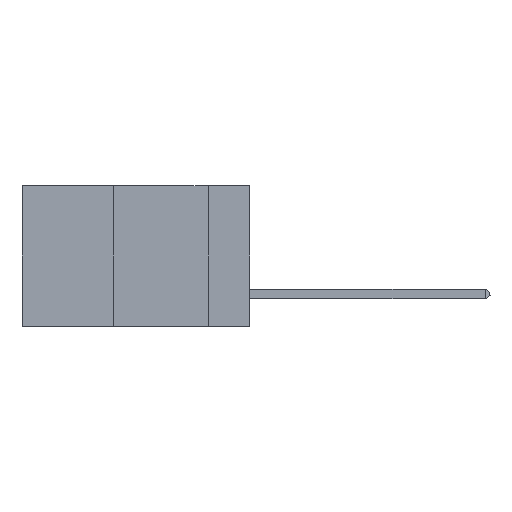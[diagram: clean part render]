
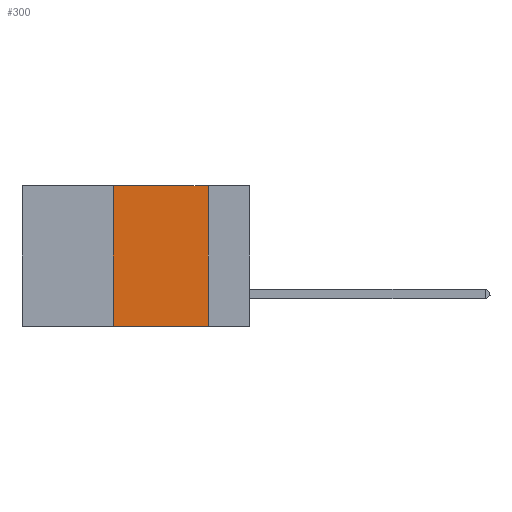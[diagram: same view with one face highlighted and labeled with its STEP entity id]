
A CAD part, left-side view. The second image highlights one B-rep face of the part: STEP entity #300.
In plain terms, the highlighted planar face has unit normal (-1, 0, 0).
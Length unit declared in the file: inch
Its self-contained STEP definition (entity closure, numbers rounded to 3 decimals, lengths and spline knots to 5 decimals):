
#300 = ADVANCED_FACE ( 'NONE', ( #12307 ), #6551, .F. ) ;
#462 = VECTOR ( 'NONE', #12837, 39.37008 ) ;
#1482 = CARTESIAN_POINT ( 'NONE',  ( 0., 0.6, -0.37 ) ) ;
#1737 = EDGE_CURVE ( 'NONE', #7303, #14217, #5719, .T. ) ;
#1959 = LINE ( 'NONE', #15083, #2865 ) ;
#2007 = VERTEX_POINT ( 'NONE', #3994 ) ;
#2865 = VECTOR ( 'NONE', #3869, 39.37008 ) ;
#3311 = ORIENTED_EDGE ( 'NONE', *, *, #9573, .F. ) ;
#3869 = DIRECTION ( 'NONE',  ( 0., -1., 0. ) ) ;
#3994 = CARTESIAN_POINT ( 'NONE',  ( 0., 0.36, 0. ) ) ;
#4068 = VECTOR ( 'NONE', #8463, 39.37008 ) ;
#4464 = ORIENTED_EDGE ( 'NONE', *, *, #14006, .F. ) ;
#4720 = CARTESIAN_POINT ( 'NONE',  ( 0., 0.11, 0. ) ) ;
#4928 = CARTESIAN_POINT ( 'NONE',  ( 0., 0.36, -0.37 ) ) ;
#5378 = DIRECTION ( 'NONE',  ( 0., 0., -1. ) ) ;
#5719 = LINE ( 'NONE', #1482, #4068 ) ;
#6551 = PLANE ( 'NONE',  #12454 ) ;
#7303 = VERTEX_POINT ( 'NONE', #4928 ) ;
#8110 = VECTOR ( 'NONE', #13429, 39.37008 ) ;
#8463 = DIRECTION ( 'NONE',  ( 0., -1., 0. ) ) ;
#9234 = LINE ( 'NONE', #4720, #462 ) ;
#9573 = EDGE_CURVE ( 'NONE', #10202, #14217, #9234, .T. ) ;
#9601 = CARTESIAN_POINT ( 'NONE',  ( 0., 0.11, 0. ) ) ;
#10129 = DIRECTION ( 'NONE',  ( 1., 0., 0. ) ) ;
#10202 = VERTEX_POINT ( 'NONE', #9601 ) ;
#12307 = FACE_OUTER_BOUND ( 'NONE', #13466, .T. ) ;
#12454 = AXIS2_PLACEMENT_3D ( 'NONE', #14791, #10129, #5378 ) ;
#12837 = DIRECTION ( 'NONE',  ( 0., 0., -1. ) ) ;
#12965 = CARTESIAN_POINT ( 'NONE',  ( 0., 0.11, -0.37 ) ) ;
#13429 = DIRECTION ( 'NONE',  ( 0., 0., 1. ) ) ;
#13440 = ORIENTED_EDGE ( 'NONE', *, *, #13870, .F. ) ;
#13466 = EDGE_LOOP ( 'NONE', ( #3311, #4464, #13440, #14483 ) ) ;
#13870 = EDGE_CURVE ( 'NONE', #7303, #2007, #15010, .T. ) ;
#14006 = EDGE_CURVE ( 'NONE', #2007, #10202, #1959, .T. ) ;
#14217 = VERTEX_POINT ( 'NONE', #12965 ) ;
#14483 = ORIENTED_EDGE ( 'NONE', *, *, #1737, .T. ) ;
#14754 = CARTESIAN_POINT ( 'NONE',  ( 0., 0.36, 0. ) ) ;
#14791 = CARTESIAN_POINT ( 'NONE',  ( 0., 0.6, 0. ) ) ;
#15010 = LINE ( 'NONE', #14754, #8110 ) ;
#15083 = CARTESIAN_POINT ( 'NONE',  ( 0., 0.6, 0. ) ) ;
